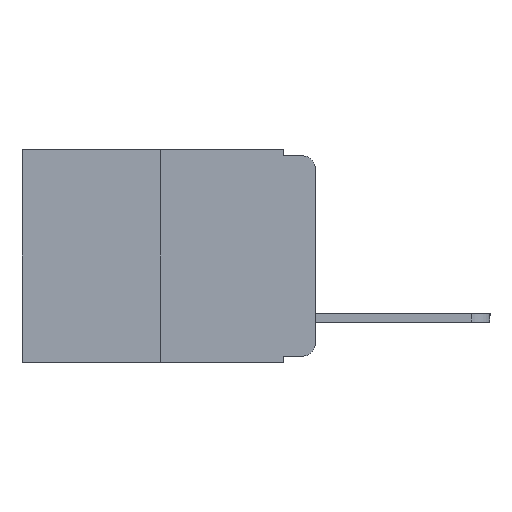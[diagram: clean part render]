
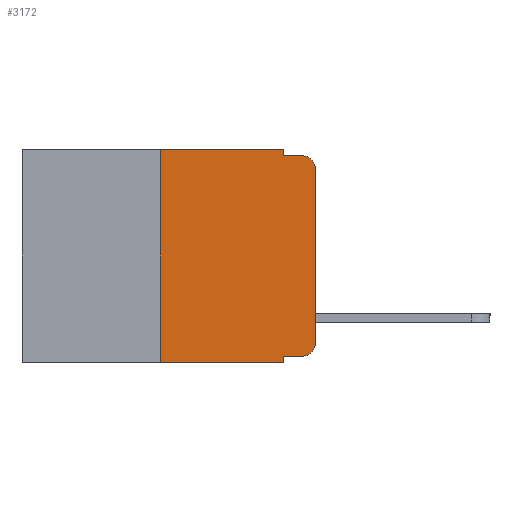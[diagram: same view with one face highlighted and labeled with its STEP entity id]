
A CAD part, left-side view. The second image highlights one B-rep face of the part: STEP entity #3172.
In plain terms, the highlighted planar face has unit normal (-1, 0, 0).
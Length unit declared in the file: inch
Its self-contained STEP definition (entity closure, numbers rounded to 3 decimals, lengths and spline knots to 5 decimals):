
#143 = CARTESIAN_POINT ( 'NONE',  ( 0., 0.051, -0.01 ) ) ;
#145 = ORIENTED_EDGE ( 'NONE', *, *, #2900, .F. ) ;
#279 = VERTEX_POINT ( 'NONE', #9056 ) ;
#299 = CARTESIAN_POINT ( 'NONE',  ( 0., 0.25, 0. ) ) ;
#563 = ORIENTED_EDGE ( 'NONE', *, *, #11478, .T. ) ;
#709 = CARTESIAN_POINT ( 'NONE',  ( 0., 0., 0. ) ) ;
#731 = ORIENTED_EDGE ( 'NONE', *, *, #1498, .T. ) ;
#867 = ORIENTED_EDGE ( 'NONE', *, *, #4993, .T. ) ;
#903 = DIRECTION ( 'NONE',  ( 0., -1., 0. ) ) ;
#1213 = CARTESIAN_POINT ( 'NONE',  ( 0., 0.051, -0.333 ) ) ;
#1392 = EDGE_CURVE ( 'NONE', #2283, #2978, #4541, .T. ) ;
#1463 = CARTESIAN_POINT ( 'NONE',  ( 0., 0.051, 0. ) ) ;
#1498 = EDGE_CURVE ( 'NONE', #4396, #3327, #2394, .T. ) ;
#1682 = ORIENTED_EDGE ( 'NONE', *, *, #5309, .F. ) ;
#1835 = VECTOR ( 'NONE', #8861, 39.37008 ) ;
#2066 = ORIENTED_EDGE ( 'NONE', *, *, #5525, .F. ) ;
#2147 = VERTEX_POINT ( 'NONE', #6751 ) ;
#2157 = ORIENTED_EDGE ( 'NONE', *, *, #3528, .F. ) ;
#2283 = VERTEX_POINT ( 'NONE', #11318 ) ;
#2394 = CIRCLE ( 'NONE', #5179, 0.02 ) ;
#2411 = DIRECTION ( 'NONE',  ( 0., -1., 0. ) ) ;
#2681 = VECTOR ( 'NONE', #8401, 39.37008 ) ;
#2725 = LINE ( 'NONE', #1213, #8240 ) ;
#2866 = VERTEX_POINT ( 'NONE', #143 ) ;
#2900 = EDGE_CURVE ( 'NONE', #2147, #2978, #6148, .T. ) ;
#2978 = VERTEX_POINT ( 'NONE', #13062 ) ;
#3172 = ADVANCED_FACE ( 'NONE', ( #6796 ), #8936, .F. ) ;
#3327 = VERTEX_POINT ( 'NONE', #8324 ) ;
#3528 = EDGE_CURVE ( 'NONE', #10172, #7820, #13479, .T. ) ;
#3542 = DIRECTION ( 'NONE',  ( 0., 0., -1. ) ) ;
#3556 = VECTOR ( 'NONE', #8533, 39.37008 ) ;
#3628 = DIRECTION ( 'NONE',  ( 0., 0., -1. ) ) ;
#4256 = CARTESIAN_POINT ( 'NONE',  ( 0., 0.02, -0.03 ) ) ;
#4396 = VERTEX_POINT ( 'NONE', #7475 ) ;
#4541 = LINE ( 'NONE', #10357, #1835 ) ;
#4587 = EDGE_LOOP ( 'NONE', ( #8114, #867, #1682, #2066, #2157, #7265, #8313, #145, #563, #731 ) ) ;
#4648 = CARTESIAN_POINT ( 'NONE',  ( 0., 0.473, 0. ) ) ;
#4834 = EDGE_CURVE ( 'NONE', #2283, #10172, #11577, .T. ) ;
#4987 = EDGE_CURVE ( 'NONE', #3327, #279, #8967, .T. ) ;
#4993 = EDGE_CURVE ( 'NONE', #279, #7099, #11431, .T. ) ;
#5179 = AXIS2_PLACEMENT_3D ( 'NONE', #9276, #9557, #13465 ) ;
#5309 = EDGE_CURVE ( 'NONE', #2866, #7099, #5756, .T. ) ;
#5435 = DIRECTION ( 'NONE',  ( 0., 0., -1. ) ) ;
#5525 = EDGE_CURVE ( 'NONE', #7820, #2866, #12718, .T. ) ;
#5527 = CARTESIAN_POINT ( 'NONE',  ( 0., 0.25, 0. ) ) ;
#5756 = LINE ( 'NONE', #9396, #2681 ) ;
#6122 = VECTOR ( 'NONE', #903, 39.37008 ) ;
#6148 = LINE ( 'NONE', #1463, #13498 ) ;
#6751 = CARTESIAN_POINT ( 'NONE',  ( 0., 0.051, -0.333 ) ) ;
#6796 = FACE_OUTER_BOUND ( 'NONE', #4587, .T. ) ;
#7099 = VERTEX_POINT ( 'NONE', #11203 ) ;
#7155 = DIRECTION ( 'NONE',  ( 0., 0., -1. ) ) ;
#7265 = ORIENTED_EDGE ( 'NONE', *, *, #4834, .F. ) ;
#7475 = CARTESIAN_POINT ( 'NONE',  ( 0., 0.02, -0.333 ) ) ;
#7715 = VECTOR ( 'NONE', #3628, 39.37008 ) ;
#7820 = VERTEX_POINT ( 'NONE', #11605 ) ;
#8114 = ORIENTED_EDGE ( 'NONE', *, *, #4987, .T. ) ;
#8222 = DIRECTION ( 'NONE',  ( 0., 0., 1. ) ) ;
#8240 = VECTOR ( 'NONE', #2411, 39.37008 ) ;
#8313 = ORIENTED_EDGE ( 'NONE', *, *, #1392, .T. ) ;
#8324 = CARTESIAN_POINT ( 'NONE',  ( 0., 0., -0.313 ) ) ;
#8401 = DIRECTION ( 'NONE',  ( 0., -1., 0. ) ) ;
#8533 = DIRECTION ( 'NONE',  ( 0., 0., 1. ) ) ;
#8690 = CARTESIAN_POINT ( 'NONE',  ( 0., 0.473, 0. ) ) ;
#8861 = DIRECTION ( 'NONE',  ( 0., -1., 0. ) ) ;
#8936 = PLANE ( 'NONE',  #10585 ) ;
#8967 = LINE ( 'NONE', #709, #3556 ) ;
#9056 = CARTESIAN_POINT ( 'NONE',  ( 0., 0., -0.03 ) ) ;
#9276 = CARTESIAN_POINT ( 'NONE',  ( 0., 0.02, -0.313 ) ) ;
#9396 = CARTESIAN_POINT ( 'NONE',  ( 0., 0.051, -0.01 ) ) ;
#9429 = VECTOR ( 'NONE', #8222, 39.37008 ) ;
#9557 = DIRECTION ( 'NONE',  ( -1., 0., 0. ) ) ;
#9910 = DIRECTION ( 'NONE',  ( 1., 0., 0. ) ) ;
#9975 = CARTESIAN_POINT ( 'NONE',  ( 0., 0.051, 0. ) ) ;
#10172 = VERTEX_POINT ( 'NONE', #5527 ) ;
#10357 = CARTESIAN_POINT ( 'NONE',  ( 0., 0.473, -0.343 ) ) ;
#10585 = AXIS2_PLACEMENT_3D ( 'NONE', #4648, #9910, #3542 ) ;
#10905 = AXIS2_PLACEMENT_3D ( 'NONE', #4256, #11369, #5435 ) ;
#11203 = CARTESIAN_POINT ( 'NONE',  ( 0., 0.02, -0.01 ) ) ;
#11318 = CARTESIAN_POINT ( 'NONE',  ( 0., 0.25, -0.343 ) ) ;
#11369 = DIRECTION ( 'NONE',  ( -1., 0., 0. ) ) ;
#11431 = CIRCLE ( 'NONE', #10905, 0.02 ) ;
#11478 = EDGE_CURVE ( 'NONE', #2147, #4396, #2725, .T. ) ;
#11577 = LINE ( 'NONE', #299, #9429 ) ;
#11605 = CARTESIAN_POINT ( 'NONE',  ( 0., 0.051, 0. ) ) ;
#12718 = LINE ( 'NONE', #9975, #7715 ) ;
#13062 = CARTESIAN_POINT ( 'NONE',  ( 0., 0.051, -0.343 ) ) ;
#13465 = DIRECTION ( 'NONE',  ( 0., 0., -1. ) ) ;
#13479 = LINE ( 'NONE', #8690, #6122 ) ;
#13498 = VECTOR ( 'NONE', #7155, 39.37008 ) ;
